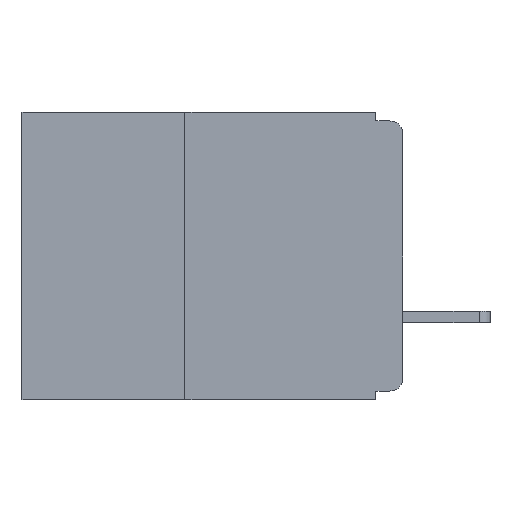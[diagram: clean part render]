
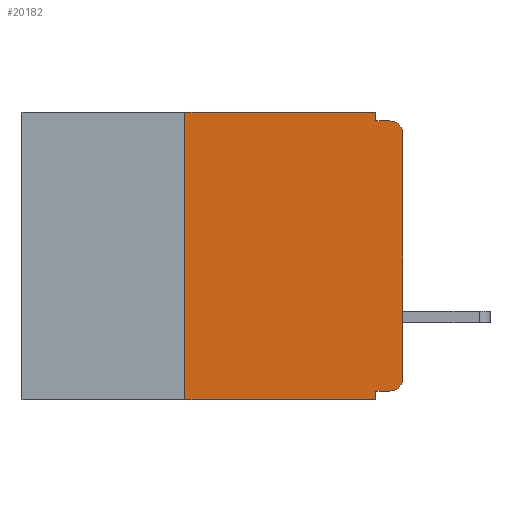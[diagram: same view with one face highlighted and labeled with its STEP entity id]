
A CAD part, left-side view. The second image highlights one B-rep face of the part: STEP entity #20182.
In plain terms, the highlighted planar face has unit normal (-1, 0, 0).
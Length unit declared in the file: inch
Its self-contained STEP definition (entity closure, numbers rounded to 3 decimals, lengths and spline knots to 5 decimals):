
#553 = DIRECTION ( 'NONE',  ( 0., 0., -1. ) ) ;
#590 = EDGE_CURVE ( 'NONE', #14979, #20951, #7249, .T. ) ;
#1408 = VECTOR ( 'NONE', #18362, 39.37008 ) ;
#1410 = VECTOR ( 'NONE', #22143, 39.37008 ) ;
#2030 = LINE ( 'NONE', #11376, #2719 ) ;
#2719 = VECTOR ( 'NONE', #11309, 39.37008 ) ;
#2774 = DIRECTION ( 'NONE',  ( 0., 0., 1. ) ) ;
#2792 = ORIENTED_EDGE ( 'NONE', *, *, #5186, .F. ) ;
#3486 = CIRCLE ( 'NONE', #6111, 0.015 ) ;
#3585 = ORIENTED_EDGE ( 'NONE', *, *, #15168, .F. ) ;
#4000 = EDGE_CURVE ( 'NONE', #16024, #14979, #2030, .T. ) ;
#4157 = ORIENTED_EDGE ( 'NONE', *, *, #13283, .T. ) ;
#4262 = DIRECTION ( 'NONE',  ( 0., 0., -1. ) ) ;
#4287 = DIRECTION ( 'NONE',  ( -1., 0., 0. ) ) ;
#4312 = CARTESIAN_POINT ( 'NONE',  ( 0., 0.015, -0.305 ) ) ;
#4709 = VECTOR ( 'NONE', #15337, 39.37008 ) ;
#5186 = EDGE_CURVE ( 'NONE', #20951, #26226, #9771, .T. ) ;
#5201 = DIRECTION ( 'NONE',  ( -1., 0., 0. ) ) ;
#5210 = DIRECTION ( 'NONE',  ( 0., 0., 1. ) ) ;
#5637 = VERTEX_POINT ( 'NONE', #9111 ) ;
#5722 = VECTOR ( 'NONE', #5210, 39.37008 ) ;
#6111 = AXIS2_PLACEMENT_3D ( 'NONE', #4312, #4287, #4262 ) ;
#6466 = LINE ( 'NONE', #18337, #27461 ) ;
#6478 = VERTEX_POINT ( 'NONE', #20808 ) ;
#6646 = DIRECTION ( 'NONE',  ( 1., 0., 0. ) ) ;
#7179 = VERTEX_POINT ( 'NONE', #25304 ) ;
#7189 = ORIENTED_EDGE ( 'NONE', *, *, #25845, .T. ) ;
#7249 = LINE ( 'NONE', #10020, #1410 ) ;
#7711 = EDGE_CURVE ( 'NONE', #22563, #6478, #23375, .T. ) ;
#8446 = CARTESIAN_POINT ( 'NONE',  ( 0., 0.031, -0.33 ) ) ;
#8738 = EDGE_CURVE ( 'NONE', #22563, #5637, #3486, .T. ) ;
#9049 = FACE_OUTER_BOUND ( 'NONE', #18126, .T. ) ;
#9111 = CARTESIAN_POINT ( 'NONE',  ( 0., 0., -0.305 ) ) ;
#9771 = LINE ( 'NONE', #15397, #4709 ) ;
#9977 = DIRECTION ( 'NONE',  ( 0., -1., 0. ) ) ;
#10020 = CARTESIAN_POINT ( 'NONE',  ( 0., 0.031, 0. ) ) ;
#10338 = ORIENTED_EDGE ( 'NONE', *, *, #19478, .F. ) ;
#10369 = CARTESIAN_POINT ( 'NONE',  ( 0., 0.25, 0. ) ) ;
#11309 = DIRECTION ( 'NONE',  ( 0., -1., 0. ) ) ;
#11376 = CARTESIAN_POINT ( 'NONE',  ( 0., 0.437, 0. ) ) ;
#11410 = CARTESIAN_POINT ( 'NONE',  ( 0., 0., 0. ) ) ;
#11448 = CARTESIAN_POINT ( 'NONE',  ( 0., 0.031, -0.33 ) ) ;
#11546 = AXIS2_PLACEMENT_3D ( 'NONE', #14105, #6646, #21405 ) ;
#13283 = EDGE_CURVE ( 'NONE', #19607, #26226, #25375, .T. ) ;
#13361 = AXIS2_PLACEMENT_3D ( 'NONE', #17932, #5201, #20006 ) ;
#14105 = CARTESIAN_POINT ( 'NONE',  ( 0., 0.437, 0. ) ) ;
#14869 = CARTESIAN_POINT ( 'NONE',  ( 0., 0.031, 0. ) ) ;
#14979 = VERTEX_POINT ( 'NONE', #14869 ) ;
#15168 = EDGE_CURVE ( 'NONE', #6478, #21979, #20051, .T. ) ;
#15337 = DIRECTION ( 'NONE',  ( 0., -1., 0. ) ) ;
#15397 = CARTESIAN_POINT ( 'NONE',  ( 0., 0., -0.01 ) ) ;
#16024 = VERTEX_POINT ( 'NONE', #10369 ) ;
#16533 = EDGE_CURVE ( 'NONE', #7179, #21979, #6466, .T. ) ;
#17852 = ORIENTED_EDGE ( 'NONE', *, *, #590, .F. ) ;
#17932 = CARTESIAN_POINT ( 'NONE',  ( 0., 0.015, -0.025 ) ) ;
#17939 = CARTESIAN_POINT ( 'NONE',  ( 0., 0.25, -0.33 ) ) ;
#18126 = EDGE_LOOP ( 'NONE', ( #7189, #4157, #2792, #17852, #18235, #10338, #22793, #3585, #19544, #24770 ) ) ;
#18235 = ORIENTED_EDGE ( 'NONE', *, *, #4000, .F. ) ;
#18304 = CARTESIAN_POINT ( 'NONE',  ( 0., 0., -0.025 ) ) ;
#18337 = CARTESIAN_POINT ( 'NONE',  ( 0., 0.437, -0.33 ) ) ;
#18362 = DIRECTION ( 'NONE',  ( 0., 1., 0. ) ) ;
#18453 = CARTESIAN_POINT ( 'NONE',  ( 0., 0., -0.32 ) ) ;
#19392 = VECTOR ( 'NONE', #553, 39.37008 ) ;
#19478 = EDGE_CURVE ( 'NONE', #7179, #16024, #26763, .T. ) ;
#19544 = ORIENTED_EDGE ( 'NONE', *, *, #7711, .F. ) ;
#19607 = VERTEX_POINT ( 'NONE', #18304 ) ;
#20006 = DIRECTION ( 'NONE',  ( 0., 0., -1. ) ) ;
#20051 = LINE ( 'NONE', #11448, #19392 ) ;
#20182 = ADVANCED_FACE ( 'NONE', ( #9049 ), #22363, .F. ) ;
#20808 = CARTESIAN_POINT ( 'NONE',  ( 0., 0.031, -0.32 ) ) ;
#20951 = VERTEX_POINT ( 'NONE', #23729 ) ;
#21192 = VECTOR ( 'NONE', #2774, 39.37008 ) ;
#21405 = DIRECTION ( 'NONE',  ( 0., 0., -1. ) ) ;
#21830 = LINE ( 'NONE', #11410, #21192 ) ;
#21979 = VERTEX_POINT ( 'NONE', #8446 ) ;
#22143 = DIRECTION ( 'NONE',  ( 0., 0., -1. ) ) ;
#22363 = PLANE ( 'NONE',  #11546 ) ;
#22563 = VERTEX_POINT ( 'NONE', #25441 ) ;
#22793 = ORIENTED_EDGE ( 'NONE', *, *, #16533, .T. ) ;
#23375 = LINE ( 'NONE', #18453, #1408 ) ;
#23729 = CARTESIAN_POINT ( 'NONE',  ( 0., 0.031, -0.01 ) ) ;
#24770 = ORIENTED_EDGE ( 'NONE', *, *, #8738, .T. ) ;
#25237 = CARTESIAN_POINT ( 'NONE',  ( 0., 0.015, -0.01 ) ) ;
#25304 = CARTESIAN_POINT ( 'NONE',  ( 0., 0.25, -0.33 ) ) ;
#25375 = CIRCLE ( 'NONE', #13361, 0.015 ) ;
#25441 = CARTESIAN_POINT ( 'NONE',  ( 0., 0.015, -0.32 ) ) ;
#25845 = EDGE_CURVE ( 'NONE', #5637, #19607, #21830, .T. ) ;
#26226 = VERTEX_POINT ( 'NONE', #25237 ) ;
#26763 = LINE ( 'NONE', #17939, #5722 ) ;
#27461 = VECTOR ( 'NONE', #9977, 39.37008 ) ;
